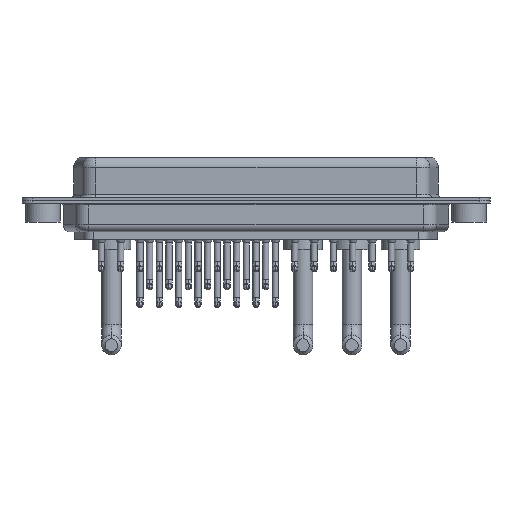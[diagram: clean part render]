
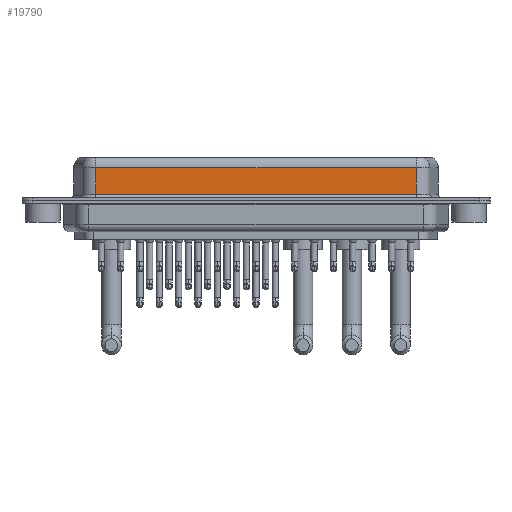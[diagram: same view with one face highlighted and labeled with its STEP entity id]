
A CAD part, front view. The second image highlights one B-rep face of the part: STEP entity #19790.
In plain terms, the highlighted planar face has unit normal (0, -1, 0).
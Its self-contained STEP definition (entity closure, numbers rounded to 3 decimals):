
#262 = ORIENTED_EDGE ( 'NONE', *, *, #7822, .T. ) ;
#499 = CARTESIAN_POINT ( 'NONE',  ( 7.59, -5.375, 6.4 ) ) ;
#2129 = LINE ( 'NONE', #499, #5798 ) ;
#2836 = VERTEX_POINT ( 'NONE', #18971 ) ;
#3405 = DIRECTION ( 'NONE',  ( -1., 0., 0. ) ) ;
#4067 = DIRECTION ( 'NONE',  ( 1., 0., 0. ) ) ;
#4456 = EDGE_CURVE ( 'NONE', #2836, #20535, #2129, .T. ) ;
#4649 = DIRECTION ( 'NONE',  ( 0., 0., -1. ) ) ;
#4677 = ORIENTED_EDGE ( 'NONE', *, *, #14622, .F. ) ;
#4758 = ORIENTED_EDGE ( 'NONE', *, *, #25069, .T. ) ;
#5798 = VECTOR ( 'NONE', #4649, 1000. ) ;
#6434 = LINE ( 'NONE', #15429, #27240 ) ;
#6721 = DIRECTION ( 'NONE',  ( 0., 1., 0. ) ) ;
#6853 = DIRECTION ( 'NONE',  ( 0., 0., 1. ) ) ;
#7697 = VERTEX_POINT ( 'NONE', #28108 ) ;
#7822 = EDGE_CURVE ( 'NONE', #20535, #23535, #6434, .T. ) ;
#9147 = CARTESIAN_POINT ( 'NONE',  ( 53.41, -5.375, 0.9 ) ) ;
#10300 = ORIENTED_EDGE ( 'NONE', *, *, #4456, .T. ) ;
#11565 = VECTOR ( 'NONE', #3405, 1000. ) ;
#14622 = EDGE_CURVE ( 'NONE', #7697, #23535, #19665, .T. ) ;
#14926 = VECTOR ( 'NONE', #22320, 1000. ) ;
#15429 = CARTESIAN_POINT ( 'NONE',  ( 53.41, -5.375, 0.9 ) ) ;
#16017 = CARTESIAN_POINT ( 'NONE',  ( 53.41, -5.375, 6.4 ) ) ;
#16123 = AXIS2_PLACEMENT_3D ( 'NONE', #16017, #6721, #6853 ) ;
#16709 = CARTESIAN_POINT ( 'NONE',  ( 7.59, -5.375, 0.9 ) ) ;
#18238 = PLANE ( 'NONE',  #16123 ) ;
#18776 = LINE ( 'NONE', #23674, #11565 ) ;
#18784 = EDGE_LOOP ( 'NONE', ( #4677, #4758, #10300, #262 ) ) ;
#18971 = CARTESIAN_POINT ( 'NONE',  ( 7.59, -5.375, 4.65 ) ) ;
#19665 = LINE ( 'NONE', #24410, #14926 ) ;
#19790 = ADVANCED_FACE ( 'NONE', ( #25087 ), #18238, .F. ) ;
#20535 = VERTEX_POINT ( 'NONE', #16709 ) ;
#22320 = DIRECTION ( 'NONE',  ( 0., 0., -1. ) ) ;
#23535 = VERTEX_POINT ( 'NONE', #9147 ) ;
#23674 = CARTESIAN_POINT ( 'NONE',  ( 53.41, -5.375, 4.65 ) ) ;
#24410 = CARTESIAN_POINT ( 'NONE',  ( 53.41, -5.375, 6.4 ) ) ;
#25069 = EDGE_CURVE ( 'NONE', #7697, #2836, #18776, .T. ) ;
#25087 = FACE_OUTER_BOUND ( 'NONE', #18784, .T. ) ;
#27240 = VECTOR ( 'NONE', #4067, 1000. ) ;
#28108 = CARTESIAN_POINT ( 'NONE',  ( 53.41, -5.375, 4.65 ) ) ;
